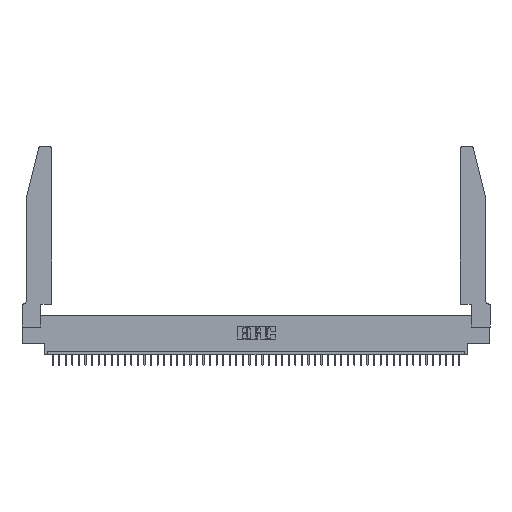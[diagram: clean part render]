
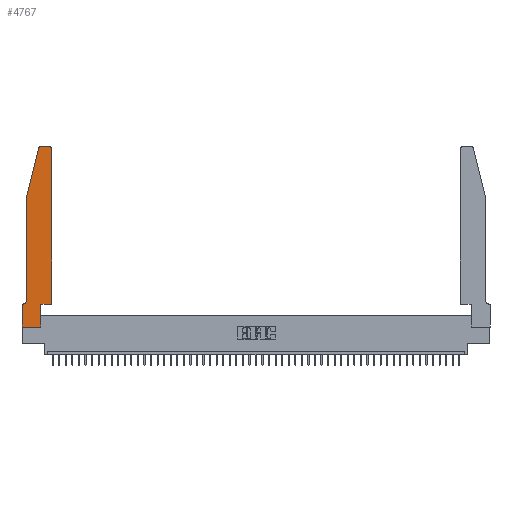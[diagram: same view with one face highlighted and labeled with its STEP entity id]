
A CAD part, top view. The second image highlights one B-rep face of the part: STEP entity #4767.
In plain terms, the highlighted planar face has unit normal (0, 0, 1).
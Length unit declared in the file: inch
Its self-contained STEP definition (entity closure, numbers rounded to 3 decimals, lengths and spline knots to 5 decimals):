
#458 = LINE ( 'NONE', #25416, #26850 ) ;
#1968 = DIRECTION ( 'NONE',  ( 0., -1., 0. ) ) ;
#2083 = VERTEX_POINT ( 'NONE', #47523 ) ;
#2982 = CARTESIAN_POINT ( 'NONE',  ( 0.4505, 0.35, 0.37 ) ) ;
#3566 = EDGE_CURVE ( 'NONE', #36636, #2083, #39537, .T. ) ;
#4101 = CARTESIAN_POINT ( 'NONE',  ( 0.284, 2.72, 0.37 ) ) ;
#4767 = ADVANCED_FACE ( 'NONE', ( #37595 ), #26141, .T. ) ;
#6809 = ORIENTED_EDGE ( 'NONE', *, *, #23644, .T. ) ;
#6835 = CIRCLE ( 'NONE', #25423, 0.07 ) ;
#8888 = EDGE_CURVE ( 'NONE', #2083, #18785, #458, .T. ) ;
#8963 = ORIENTED_EDGE ( 'NONE', *, *, #3566, .T. ) ;
#9028 = CARTESIAN_POINT ( 'NONE',  ( 0.4505, 0.35, 0.37 ) ) ;
#9598 = EDGE_CURVE ( 'NONE', #34484, #30139, #45972, .T. ) ;
#9743 = VERTEX_POINT ( 'NONE', #24347 ) ;
#10371 = VECTOR ( 'NONE', #28499, 39.37008 ) ;
#10540 = VECTOR ( 'NONE', #43818, 39.37008 ) ;
#11602 = CARTESIAN_POINT ( 'NONE',  ( 0.0055, 0.42, 0.37 ) ) ;
#11791 = LINE ( 'NONE', #24513, #16609 ) ;
#12591 = LINE ( 'NONE', #33962, #42690 ) ;
#12681 = EDGE_LOOP ( 'NONE', ( #14461, #35526, #6809, #35797, #26816, #8963, #28102, #33464, #30488, #35885, #42449, #47382 ) ) ;
#12824 = DIRECTION ( 'NONE',  ( 1., 0., 0. ) ) ;
#12895 = EDGE_CURVE ( 'NONE', #30139, #13032, #25387, .T. ) ;
#13032 = VERTEX_POINT ( 'NONE', #9028 ) ;
#13210 = LINE ( 'NONE', #29703, #49198 ) ;
#13479 = CARTESIAN_POINT ( 'NONE',  ( 0., 0., 0.37 ) ) ;
#14461 = ORIENTED_EDGE ( 'NONE', *, *, #21825, .T. ) ;
#15329 = DIRECTION ( 'NONE',  ( 0., 0., -1. ) ) ;
#15718 = LINE ( 'NONE', #33019, #10371 ) ;
#16609 = VECTOR ( 'NONE', #35537, 39.37008 ) ;
#17455 = EDGE_CURVE ( 'NONE', #18785, #34484, #28506, .T. ) ;
#18785 = VERTEX_POINT ( 'NONE', #13479 ) ;
#19049 = CARTESIAN_POINT ( 'NONE',  ( 0.2865, 0.35, 0.37 ) ) ;
#20667 = VERTEX_POINT ( 'NONE', #25233 ) ;
#21225 = EDGE_CURVE ( 'NONE', #9743, #34527, #13210, .T. ) ;
#21825 = EDGE_CURVE ( 'NONE', #20667, #31087, #12591, .T. ) ;
#22114 = DIRECTION ( 'NONE',  ( 1., 0., 0. ) ) ;
#22856 = CARTESIAN_POINT ( 'NONE',  ( 0.4505, 2.72, 0.37 ) ) ;
#23644 = EDGE_CURVE ( 'NONE', #24160, #9743, #11791, .T. ) ;
#23754 = DIRECTION ( 'NONE',  ( -1., 0., 0. ) ) ;
#24160 = VERTEX_POINT ( 'NONE', #27841 ) ;
#24347 = CARTESIAN_POINT ( 'NONE',  ( 0.0755, 2., 0.37 ) ) ;
#24513 = CARTESIAN_POINT ( 'NONE',  ( 0.0755, 2., 0.37 ) ) ;
#25233 = CARTESIAN_POINT ( 'NONE',  ( 0.4205, 2.75, 0.37 ) ) ;
#25387 = LINE ( 'NONE', #2982, #43949 ) ;
#25416 = CARTESIAN_POINT ( 'NONE',  ( 0., 0., 0.37 ) ) ;
#25423 = AXIS2_PLACEMENT_3D ( 'NONE', #11602, #15329, #42197 ) ;
#25623 = EDGE_CURVE ( 'NONE', #31087, #24160, #48031, .T. ) ;
#26141 = PLANE ( 'NONE',  #48805 ) ;
#26816 = ORIENTED_EDGE ( 'NONE', *, *, #33937, .T. ) ;
#26850 = VECTOR ( 'NONE', #1968, 39.37008 ) ;
#27841 = CARTESIAN_POINT ( 'NONE',  ( 0.25487, 2.72718, 0.37 ) ) ;
#28102 = ORIENTED_EDGE ( 'NONE', *, *, #8888, .T. ) ;
#28246 = CARTESIAN_POINT ( 'NONE',  ( 0.2865, 0., 0.37 ) ) ;
#28484 = DIRECTION ( 'NONE',  ( 1., 0., 0. ) ) ;
#28499 = DIRECTION ( 'NONE',  ( 0., 1., 0. ) ) ;
#28506 = LINE ( 'NONE', #47537, #41782 ) ;
#28862 = DIRECTION ( 'NONE',  ( 1., 0., 0. ) ) ;
#29347 = VECTOR ( 'NONE', #23754, 39.37008 ) ;
#29637 = DIRECTION ( 'NONE',  ( 1., 0., 0. ) ) ;
#29703 = CARTESIAN_POINT ( 'NONE',  ( 0.0755, 2., 0.37 ) ) ;
#29874 = VERTEX_POINT ( 'NONE', #22856 ) ;
#30014 = DIRECTION ( 'NONE',  ( 0., 0., 1. ) ) ;
#30139 = VERTEX_POINT ( 'NONE', #19049 ) ;
#30488 = ORIENTED_EDGE ( 'NONE', *, *, #9598, .T. ) ;
#31087 = VERTEX_POINT ( 'NONE', #47570 ) ;
#31658 = AXIS2_PLACEMENT_3D ( 'NONE', #4101, #42030, #28484 ) ;
#32225 = CARTESIAN_POINT ( 'NONE',  ( 0.2865, 0.35, 0.37 ) ) ;
#33019 = CARTESIAN_POINT ( 'NONE',  ( 0.4505, 0.35, 0.37 ) ) ;
#33464 = ORIENTED_EDGE ( 'NONE', *, *, #17455, .T. ) ;
#33937 = EDGE_CURVE ( 'NONE', #34527, #36636, #6835, .T. ) ;
#33962 = CARTESIAN_POINT ( 'NONE',  ( 0.2605, 2.75, 0.37 ) ) ;
#34484 = VERTEX_POINT ( 'NONE', #28246 ) ;
#34527 = VERTEX_POINT ( 'NONE', #43854 ) ;
#35135 = EDGE_CURVE ( 'NONE', #29874, #20667, #42139, .T. ) ;
#35526 = ORIENTED_EDGE ( 'NONE', *, *, #25623, .T. ) ;
#35537 = DIRECTION ( 'NONE',  ( -0.239, -0.971, 0. ) ) ;
#35797 = ORIENTED_EDGE ( 'NONE', *, *, #21225, .T. ) ;
#35885 = ORIENTED_EDGE ( 'NONE', *, *, #12895, .T. ) ;
#36636 = VERTEX_POINT ( 'NONE', #38020 ) ;
#36764 = CARTESIAN_POINT ( 'NONE',  ( 0.4205, 2.72, 0.37 ) ) ;
#37595 = FACE_OUTER_BOUND ( 'NONE', #12681, .T. ) ;
#38019 = AXIS2_PLACEMENT_3D ( 'NONE', #36764, #47919, #28862 ) ;
#38020 = CARTESIAN_POINT ( 'NONE',  ( 0.0055, 0.35, 0.37 ) ) ;
#39537 = LINE ( 'NONE', #48212, #29347 ) ;
#41782 = VECTOR ( 'NONE', #12824, 39.37008 ) ;
#42030 = DIRECTION ( 'NONE',  ( 0., 0., 1. ) ) ;
#42139 = CIRCLE ( 'NONE', #38019, 0.03 ) ;
#42197 = DIRECTION ( 'NONE',  ( -1., 0., 0. ) ) ;
#42449 = ORIENTED_EDGE ( 'NONE', *, *, #46484, .T. ) ;
#42690 = VECTOR ( 'NONE', #45852, 39.37008 ) ;
#43818 = DIRECTION ( 'NONE',  ( 0., 1., 0. ) ) ;
#43854 = CARTESIAN_POINT ( 'NONE',  ( 0.0755, 0.42, 0.37 ) ) ;
#43949 = VECTOR ( 'NONE', #29637, 39.37008 ) ;
#45852 = DIRECTION ( 'NONE',  ( -1., 0., 0. ) ) ;
#45972 = LINE ( 'NONE', #32225, #10540 ) ;
#46484 = EDGE_CURVE ( 'NONE', #13032, #29874, #15718, .T. ) ;
#47004 = DIRECTION ( 'NONE',  ( 0., -1., 0. ) ) ;
#47382 = ORIENTED_EDGE ( 'NONE', *, *, #35135, .T. ) ;
#47523 = CARTESIAN_POINT ( 'NONE',  ( 0., 0.35, 0.37 ) ) ;
#47537 = CARTESIAN_POINT ( 'NONE',  ( 0., 0., 0.37 ) ) ;
#47570 = CARTESIAN_POINT ( 'NONE',  ( 0.284, 2.75, 0.37 ) ) ;
#47919 = DIRECTION ( 'NONE',  ( 0., 0., 1. ) ) ;
#48031 = CIRCLE ( 'NONE', #31658, 0.03 ) ;
#48212 = CARTESIAN_POINT ( 'NONE',  ( 0.0755, 0.35, 0.37 ) ) ;
#48712 = CARTESIAN_POINT ( 'NONE',  ( 0., 0.35, 0.37 ) ) ;
#48805 = AXIS2_PLACEMENT_3D ( 'NONE', #48712, #30014, #22114 ) ;
#49198 = VECTOR ( 'NONE', #47004, 39.37008 ) ;
